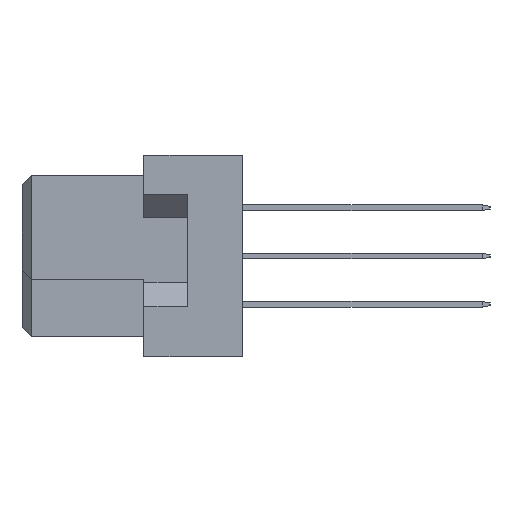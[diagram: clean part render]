
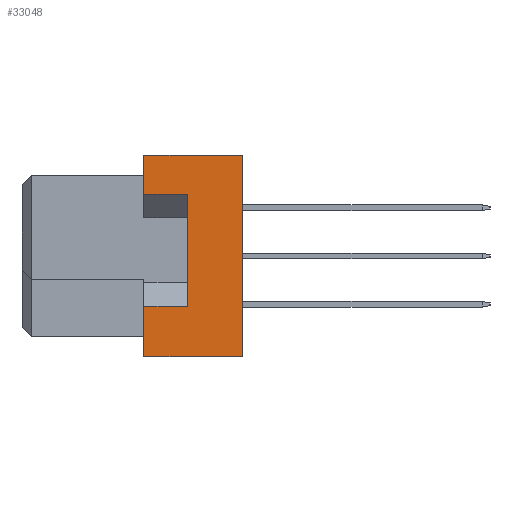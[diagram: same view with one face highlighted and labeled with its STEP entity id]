
A CAD part, left-side view. The second image highlights one B-rep face of the part: STEP entity #33048.
In plain terms, the highlighted planar face has unit normal (-1, 0, 0).
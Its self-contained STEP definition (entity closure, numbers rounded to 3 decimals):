
#398 = LINE ( 'NONE', #34710, #4607 ) ;
#622 = DIRECTION ( 'NONE',  ( 0., 0., 1. ) ) ;
#1396 = VERTEX_POINT ( 'NONE', #6864 ) ;
#1873 = CARTESIAN_POINT ( 'NONE',  ( -47.5, -6.4, -2.65 ) ) ;
#2034 = CARTESIAN_POINT ( 'NONE',  ( -47.5, -11.6, 5.3 ) ) ;
#2769 = CARTESIAN_POINT ( 'NONE',  ( -47.5, -6.4, 3.25 ) ) ;
#2901 = CARTESIAN_POINT ( 'NONE',  ( -47.5, -8.7, -2.65 ) ) ;
#3330 = ORIENTED_EDGE ( 'NONE', *, *, #12474, .F. ) ;
#4607 = VECTOR ( 'NONE', #19017, 1000. ) ;
#4658 = CARTESIAN_POINT ( 'NONE',  ( -47.5, -8.7, -2.65 ) ) ;
#5598 = VERTEX_POINT ( 'NONE', #29641 ) ;
#6714 = CARTESIAN_POINT ( 'NONE',  ( -47.5, -6.4, -5.3 ) ) ;
#6770 = CARTESIAN_POINT ( 'NONE',  ( -47.5, -11.6, 5.3 ) ) ;
#6864 = CARTESIAN_POINT ( 'NONE',  ( -47.5, -11.6, -5.3 ) ) ;
#6913 = EDGE_CURVE ( 'NONE', #1396, #16443, #17548, .T. ) ;
#7603 = LINE ( 'NONE', #23698, #26514 ) ;
#10168 = ORIENTED_EDGE ( 'NONE', *, *, #40426, .F. ) ;
#12063 = LINE ( 'NONE', #14352, #31578 ) ;
#12474 = EDGE_CURVE ( 'NONE', #31624, #19105, #36661, .T. ) ;
#13862 = CARTESIAN_POINT ( 'NONE',  ( -47.5, -11.6, 5.3 ) ) ;
#14352 = CARTESIAN_POINT ( 'NONE',  ( -47.5, -11.6, -5.3 ) ) ;
#14440 = LINE ( 'NONE', #21248, #26369 ) ;
#14966 = ORIENTED_EDGE ( 'NONE', *, *, #22416, .F. ) ;
#15750 = ORIENTED_EDGE ( 'NONE', *, *, #6913, .T. ) ;
#16443 = VERTEX_POINT ( 'NONE', #40354 ) ;
#16494 = VERTEX_POINT ( 'NONE', #2769 ) ;
#17548 = LINE ( 'NONE', #2034, #25239 ) ;
#18785 = EDGE_CURVE ( 'NONE', #1396, #24731, #12063, .T. ) ;
#18914 = LINE ( 'NONE', #6714, #40776 ) ;
#19017 = DIRECTION ( 'NONE',  ( 0., 1., 0. ) ) ;
#19105 = VERTEX_POINT ( 'NONE', #24401 ) ;
#19115 = DIRECTION ( 'NONE',  ( 0., 0., 1. ) ) ;
#19948 = EDGE_CURVE ( 'NONE', #16443, #5598, #22478, .T. ) ;
#20327 = EDGE_LOOP ( 'NONE', ( #29246, #27785, #26301, #15750, #31917, #10168, #14966, #3330 ) ) ;
#21248 = CARTESIAN_POINT ( 'NONE',  ( -47.5, -8.7, 3.25 ) ) ;
#21354 = DIRECTION ( 'NONE',  ( 0., 1., 0. ) ) ;
#21708 = VECTOR ( 'NONE', #23096, 1000. ) ;
#22239 = EDGE_CURVE ( 'NONE', #31624, #35662, #398, .T. ) ;
#22416 = EDGE_CURVE ( 'NONE', #19105, #16494, #14440, .T. ) ;
#22478 = LINE ( 'NONE', #6770, #21708 ) ;
#23096 = DIRECTION ( 'NONE',  ( 0., 1., 0. ) ) ;
#23562 = DIRECTION ( 'NONE',  ( -1., 0., 0. ) ) ;
#23698 = CARTESIAN_POINT ( 'NONE',  ( -47.5, -6.4, -5.3 ) ) ;
#24401 = CARTESIAN_POINT ( 'NONE',  ( -47.5, -8.7, 3.25 ) ) ;
#24731 = VERTEX_POINT ( 'NONE', #40533 ) ;
#24818 = FACE_OUTER_BOUND ( 'NONE', #20327, .T. ) ;
#24844 = AXIS2_PLACEMENT_3D ( 'NONE', #13862, #23562, #622 ) ;
#25239 = VECTOR ( 'NONE', #26848, 1000. ) ;
#26301 = ORIENTED_EDGE ( 'NONE', *, *, #18785, .F. ) ;
#26369 = VECTOR ( 'NONE', #39617, 1000. ) ;
#26514 = VECTOR ( 'NONE', #39581, 1000. ) ;
#26848 = DIRECTION ( 'NONE',  ( 0., 0., 1. ) ) ;
#27785 = ORIENTED_EDGE ( 'NONE', *, *, #34910, .F. ) ;
#29246 = ORIENTED_EDGE ( 'NONE', *, *, #22239, .T. ) ;
#29641 = CARTESIAN_POINT ( 'NONE',  ( -47.5, -6.4, 5.3 ) ) ;
#31578 = VECTOR ( 'NONE', #21354, 1000. ) ;
#31624 = VERTEX_POINT ( 'NONE', #2901 ) ;
#31917 = ORIENTED_EDGE ( 'NONE', *, *, #19948, .T. ) ;
#33048 = ADVANCED_FACE ( 'NONE', ( #24818 ), #35757, .T. ) ;
#33572 = DIRECTION ( 'NONE',  ( 0., 0., 1. ) ) ;
#34710 = CARTESIAN_POINT ( 'NONE',  ( -47.5, -8.7, -2.65 ) ) ;
#34910 = EDGE_CURVE ( 'NONE', #24731, #35662, #18914, .T. ) ;
#35662 = VERTEX_POINT ( 'NONE', #1873 ) ;
#35757 = PLANE ( 'NONE',  #24844 ) ;
#36661 = LINE ( 'NONE', #4658, #39219 ) ;
#39219 = VECTOR ( 'NONE', #33572, 1000. ) ;
#39581 = DIRECTION ( 'NONE',  ( 0., 0., 1. ) ) ;
#39617 = DIRECTION ( 'NONE',  ( 0., 1., 0. ) ) ;
#40354 = CARTESIAN_POINT ( 'NONE',  ( -47.5, -11.6, 5.3 ) ) ;
#40426 = EDGE_CURVE ( 'NONE', #16494, #5598, #7603, .T. ) ;
#40533 = CARTESIAN_POINT ( 'NONE',  ( -47.5, -6.4, -5.3 ) ) ;
#40776 = VECTOR ( 'NONE', #19115, 1000. ) ;
